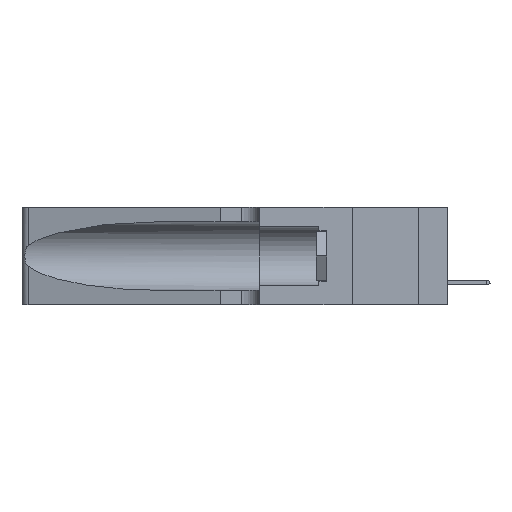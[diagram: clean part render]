
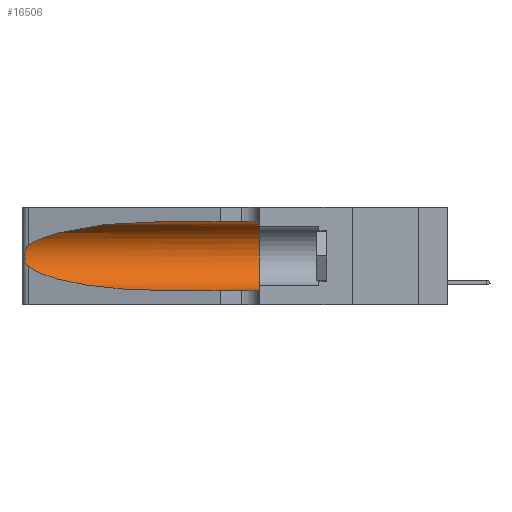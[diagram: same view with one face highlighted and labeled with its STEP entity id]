
A CAD part, left-side view. The second image highlights one B-rep face of the part: STEP entity #16506.
In plain terms, the highlighted cylindrical face has radius 3.308 mm (diameter 6.617 mm), a partial arc.
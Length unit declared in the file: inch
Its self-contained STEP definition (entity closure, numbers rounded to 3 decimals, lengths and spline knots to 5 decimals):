
#4 = CIRCLE ( 'NONE', #9742, 0.13025 ) ;
#204 = EDGE_LOOP ( 'NONE', ( #3084, #424, #12724, #15109, #17713, #10754 ) ) ;
#424 = ORIENTED_EDGE ( 'NONE', *, *, #7619, .T. ) ;
#451 = DIRECTION ( 'NONE',  ( 0., 1., 0. ) ) ;
#576 = CARTESIAN_POINT ( 'NONE',  ( 0.1305, 0.72297, 0.31525 ) ) ;
#713 = VERTEX_POINT ( 'NONE', #7797 ) ;
#967 = DIRECTION ( 'NONE',  ( 0., -1., 0. ) ) ;
#1365 = VERTEX_POINT ( 'NONE', #10716 ) ;
#1500 = CARTESIAN_POINT ( 'NONE',  ( 0.1305, 1.61858, 0.185 ) ) ;
#1565 = FACE_OUTER_BOUND ( 'NONE', #204, .T. ) ;
#1926 = VERTEX_POINT ( 'NONE', #16545 ) ;
#1944 = EDGE_CURVE ( 'NONE', #4624, #713, #10292, .T. ) ;
#2294 = VECTOR ( 'NONE', #15428, 39.37008 ) ;
#2716 = CARTESIAN_POINT ( 'NONE',  ( 0.2373, 1.15595, 0.28018 ) ) ;
#2775 =( BOUNDED_CURVE ( )  B_SPLINE_CURVE ( 3, ( #6659, #6477, #16228, #3734 ),
 .UNSPECIFIED., .F., .T. ) 
 B_SPLINE_CURVE_WITH_KNOTS ( ( 4, 4 ),
 ( 3.44316, 4.71239 ),
 .UNSPECIFIED. ) 
 CURVE ( )  GEOMETRIC_REPRESENTATION_ITEM ( )  RATIONAL_B_SPLINE_CURVE ( ( 1., 0.87, 0.87, 1. ) ) 
 REPRESENTATION_ITEM ( '' )  );
#3084 = ORIENTED_EDGE ( 'NONE', *, *, #1944, .T. ) ;
#3251 = CARTESIAN_POINT ( 'NONE',  ( 0.1305, 0.35, 0.185 ) ) ;
#3471 = CARTESIAN_POINT ( 'NONE',  ( 0.25639, 1.23186, 0.15144 ) ) ;
#3734 = CARTESIAN_POINT ( 'NONE',  ( 0.1305, 0.72297, 0.05475 ) ) ;
#4106 = CYLINDRICAL_SURFACE ( 'NONE', #16310, 0.13025 ) ;
#4237 = DIRECTION ( 'NONE',  ( 0., 0., -1. ) ) ;
#4624 = VERTEX_POINT ( 'NONE', #576 ) ;
#4786 = EDGE_CURVE ( 'NONE', #10111, #16129, #7395, .T. ) ;
#4862 = CARTESIAN_POINT ( 'NONE',  ( 0.1305, 0.72297, 0.05475 ) ) ;
#5569 = CARTESIAN_POINT ( 'NONE',  ( 0.18966, 0.96281, 0.31525 ) ) ;
#5909 = CARTESIAN_POINT ( 'NONE',  ( 0.1305, 1.61858, 0.31525 ) ) ;
#5999 = EDGE_CURVE ( 'NONE', #1926, #16129, #4, .T. ) ;
#6267 = CARTESIAN_POINT ( 'NONE',  ( 0.25787, 1.23484, 0.2124 ) ) ;
#6330 = CARTESIAN_POINT ( 'NONE',  ( 0.25555, 1.22993, 0.14849 ) ) ;
#6477 = CARTESIAN_POINT ( 'NONE',  ( 0.2373, 1.15595, 0.08982 ) ) ;
#6659 = CARTESIAN_POINT ( 'NONE',  ( 0.25487, 1.22718, 0.14631 ) ) ;
#7099 = DIRECTION ( 'NONE',  ( 0., -1., 0. ) ) ;
#7395 = LINE ( 'NONE', #10652, #8036 ) ;
#7619 = EDGE_CURVE ( 'NONE', #713, #1365, #15381, .T. ) ;
#7672 = CARTESIAN_POINT ( 'NONE',  ( 0.25789, 1.23486, 0.15765 ) ) ;
#7797 = CARTESIAN_POINT ( 'NONE',  ( 0.25487, 1.22718, 0.22369 ) ) ;
#8036 = VECTOR ( 'NONE', #967, 39.37008 ) ;
#8694 = EDGE_CURVE ( 'NONE', #4624, #1926, #16386, .T. ) ;
#8964 = CARTESIAN_POINT ( 'NONE',  ( 0.25639, 1.23184, 0.21858 ) ) ;
#9742 = AXIS2_PLACEMENT_3D ( 'NONE', #3251, #451, #15763 ) ;
#10111 = VERTEX_POINT ( 'NONE', #4862 ) ;
#10292 =( BOUNDED_CURVE ( )  B_SPLINE_CURVE ( 3, ( #14556, #5569, #2716, #10903 ),
 .UNSPECIFIED., .F., .T. ) 
 B_SPLINE_CURVE_WITH_KNOTS ( ( 4, 4 ),
 ( 1.5708, 2.84003 ),
 .UNSPECIFIED. ) 
 CURVE ( )  GEOMETRIC_REPRESENTATION_ITEM ( )  RATIONAL_B_SPLINE_CURVE ( ( 1., 0.87, 0.87, 1. ) ) 
 REPRESENTATION_ITEM ( '' )  );
#10474 = CARTESIAN_POINT ( 'NONE',  ( 0.25856, 1.23593, 0.16098 ) ) ;
#10538 = CARTESIAN_POINT ( 'NONE',  ( 0.25555, 1.22994, 0.2215 ) ) ;
#10652 = CARTESIAN_POINT ( 'NONE',  ( 0.1305, 1.61858, 0.05475 ) ) ;
#10716 = CARTESIAN_POINT ( 'NONE',  ( 0.25487, 1.22718, 0.14631 ) ) ;
#10754 = ORIENTED_EDGE ( 'NONE', *, *, #8694, .F. ) ;
#10777 = EDGE_CURVE ( 'NONE', #1365, #10111, #2775, .T. ) ;
#10903 = CARTESIAN_POINT ( 'NONE',  ( 0.25487, 1.22718, 0.22369 ) ) ;
#11792 = CARTESIAN_POINT ( 'NONE',  ( 0.26075, 1.23896, 0.178 ) ) ;
#11900 = CARTESIAN_POINT ( 'NONE',  ( 0.25487, 1.22718, 0.14631 ) ) ;
#12432 = CARTESIAN_POINT ( 'NONE',  ( 0.1305, 0.35, 0.05475 ) ) ;
#12724 = ORIENTED_EDGE ( 'NONE', *, *, #10777, .T. ) ;
#14464 = CARTESIAN_POINT ( 'NONE',  ( 0.25854, 1.2359, 0.20912 ) ) ;
#14556 = CARTESIAN_POINT ( 'NONE',  ( 0.1305, 0.72297, 0.31525 ) ) ;
#14693 = CARTESIAN_POINT ( 'NONE',  ( 0.26018, 1.23835, 0.19895 ) ) ;
#15109 = ORIENTED_EDGE ( 'NONE', *, *, #4786, .T. ) ;
#15381 = B_SPLINE_CURVE_WITH_KNOTS ( 'NONE', 3,
 ( #17363, #10538, #8964, #6267, #14464, #14693, #15974, #11792, #16031, #10474, #7672, #3471, #6330, #11900 ),
 .UNSPECIFIED., .F., .F.,
 ( 4, 2, 2, 2, 2, 2, 4 ),
 ( 0., 0.00027, 0.00053, 0.00107, 0.0016, 0.00187, 0.00214 ),
 .UNSPECIFIED. ) ;
#15428 = DIRECTION ( 'NONE',  ( 0., -1., 0. ) ) ;
#15763 = DIRECTION ( 'NONE',  ( 0., 0., 1. ) ) ;
#15974 = CARTESIAN_POINT ( 'NONE',  ( 0.26075, 1.23896, 0.19203 ) ) ;
#16031 = CARTESIAN_POINT ( 'NONE',  ( 0.26017, 1.23833, 0.17102 ) ) ;
#16129 = VERTEX_POINT ( 'NONE', #12432 ) ;
#16228 = CARTESIAN_POINT ( 'NONE',  ( 0.18966, 0.96281, 0.05475 ) ) ;
#16310 = AXIS2_PLACEMENT_3D ( 'NONE', #1500, #7099, #4237 ) ;
#16386 = LINE ( 'NONE', #5909, #2294 ) ;
#16506 = ADVANCED_FACE ( 'NONE', ( #1565 ), #4106, .F. ) ;
#16545 = CARTESIAN_POINT ( 'NONE',  ( 0.1305, 0.35, 0.31525 ) ) ;
#17363 = CARTESIAN_POINT ( 'NONE',  ( 0.25487, 1.22718, 0.22369 ) ) ;
#17713 = ORIENTED_EDGE ( 'NONE', *, *, #5999, .F. ) ;
